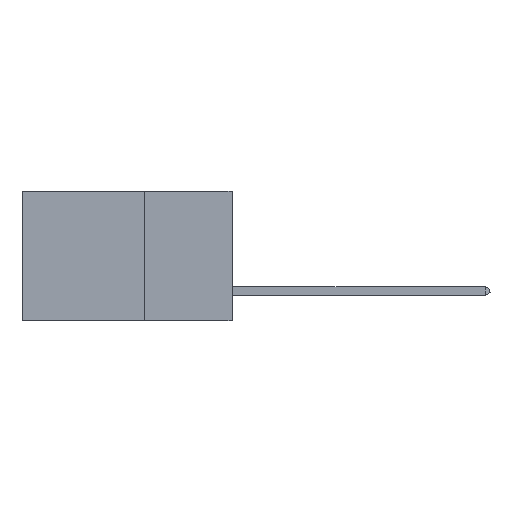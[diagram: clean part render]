
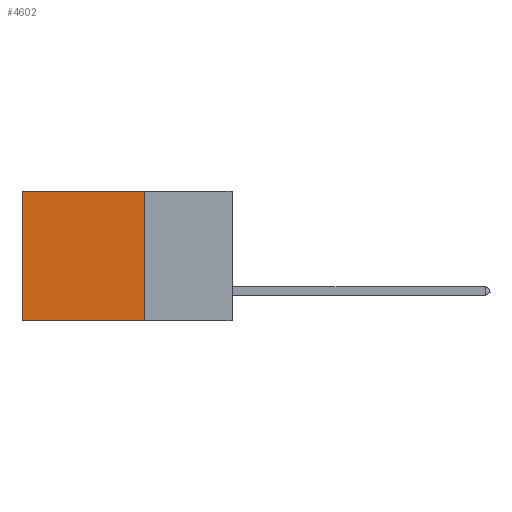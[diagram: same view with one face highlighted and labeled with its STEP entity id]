
A CAD part, left-side view. The second image highlights one B-rep face of the part: STEP entity #4602.
In plain terms, the highlighted planar face has unit normal (-1, 0, 0).
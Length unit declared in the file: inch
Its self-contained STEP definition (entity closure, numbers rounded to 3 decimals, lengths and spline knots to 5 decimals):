
#1170 = CARTESIAN_POINT ( 'NONE',  ( 0.2875, 0.25, 0. ) ) ;
#1286 = LINE ( 'NONE', #33164, #10262 ) ;
#1616 = CARTESIAN_POINT ( 'NONE',  ( 0.2875, 0.6, -0.37 ) ) ;
#2931 = LINE ( 'NONE', #42828, #38053 ) ;
#3265 = CARTESIAN_POINT ( 'NONE',  ( 0.2875, 0.6, 0. ) ) ;
#4395 = VECTOR ( 'NONE', #32172, 39.37008 ) ;
#4602 = ADVANCED_FACE ( 'NONE', ( #46546 ), #26174, .F. ) ;
#8017 = DIRECTION ( 'NONE',  ( 0., 1., 0. ) ) ;
#9522 = ORIENTED_EDGE ( 'NONE', *, *, #37353, .F. ) ;
#9763 = CARTESIAN_POINT ( 'NONE',  ( 0.2875, 0.25, 0. ) ) ;
#10262 = VECTOR ( 'NONE', #17506, 39.37008 ) ;
#10652 = ORIENTED_EDGE ( 'NONE', *, *, #40660, .F. ) ;
#11684 = EDGE_CURVE ( 'NONE', #44625, #24382, #1286, .T. ) ;
#11765 = AXIS2_PLACEMENT_3D ( 'NONE', #45159, #37661, #33349 ) ;
#12453 = CARTESIAN_POINT ( 'NONE',  ( 0.2875, 0.25, -0.37 ) ) ;
#14011 = VERTEX_POINT ( 'NONE', #1170 ) ;
#17506 = DIRECTION ( 'NONE',  ( 0., 0., -1. ) ) ;
#19106 = CARTESIAN_POINT ( 'NONE',  ( 0.2875, 0.25, -0.37 ) ) ;
#21908 = EDGE_LOOP ( 'NONE', ( #37442, #10652, #9522, #42143 ) ) ;
#24382 = VERTEX_POINT ( 'NONE', #1616 ) ;
#26174 = PLANE ( 'NONE',  #11765 ) ;
#32172 = DIRECTION ( 'NONE',  ( 0., 1., 0. ) ) ;
#33164 = CARTESIAN_POINT ( 'NONE',  ( 0.2875, 0.6, 0. ) ) ;
#33349 = DIRECTION ( 'NONE',  ( 0., 0., -1. ) ) ;
#35215 = EDGE_CURVE ( 'NONE', #14011, #44625, #47257, .T. ) ;
#37353 = EDGE_CURVE ( 'NONE', #14011, #39021, #2931, .T. ) ;
#37442 = ORIENTED_EDGE ( 'NONE', *, *, #11684, .T. ) ;
#37661 = DIRECTION ( 'NONE',  ( 1., 0., 0. ) ) ;
#38053 = VECTOR ( 'NONE', #38692, 39.37008 ) ;
#38692 = DIRECTION ( 'NONE',  ( 0., 0., -1. ) ) ;
#39021 = VERTEX_POINT ( 'NONE', #12453 ) ;
#40660 = EDGE_CURVE ( 'NONE', #39021, #24382, #47859, .T. ) ;
#42143 = ORIENTED_EDGE ( 'NONE', *, *, #35215, .T. ) ;
#42828 = CARTESIAN_POINT ( 'NONE',  ( 0.2875, 0.25, 0. ) ) ;
#44625 = VERTEX_POINT ( 'NONE', #3265 ) ;
#45159 = CARTESIAN_POINT ( 'NONE',  ( 0.2875, 0.25, 0. ) ) ;
#46546 = FACE_OUTER_BOUND ( 'NONE', #21908, .T. ) ;
#46653 = VECTOR ( 'NONE', #8017, 39.37008 ) ;
#47257 = LINE ( 'NONE', #9763, #4395 ) ;
#47859 = LINE ( 'NONE', #19106, #46653 ) ;
